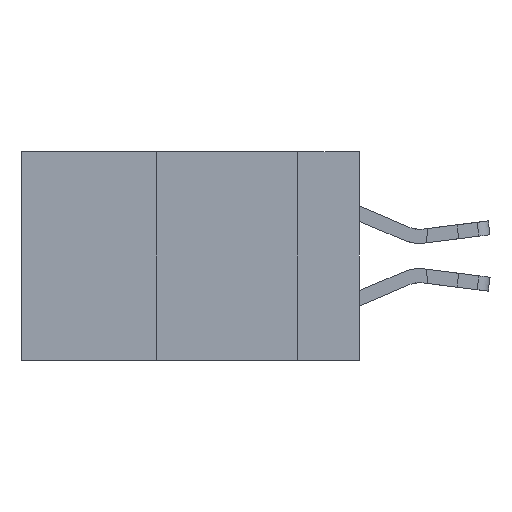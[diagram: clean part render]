
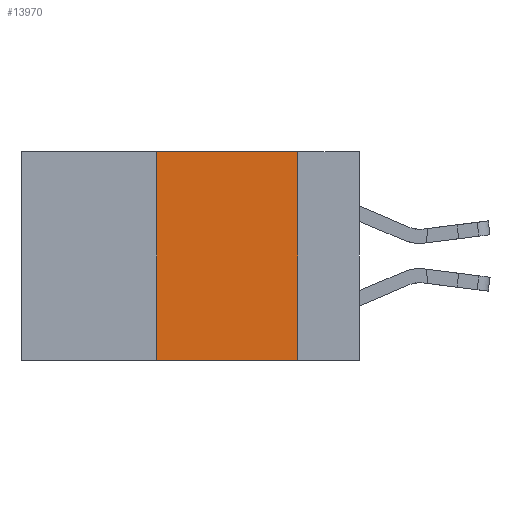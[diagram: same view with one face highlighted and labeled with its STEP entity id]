
A CAD part, left-side view. The second image highlights one B-rep face of the part: STEP entity #13970.
In plain terms, the highlighted planar face has unit normal (-1, 0, 0).
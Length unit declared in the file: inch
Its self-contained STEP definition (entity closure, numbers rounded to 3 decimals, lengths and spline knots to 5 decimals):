
#1781 = ORIENTED_EDGE ( 'NONE', *, *, #9052, .T. ) ;
#1898 = CARTESIAN_POINT ( 'NONE',  ( 0., 0.6, 0. ) ) ;
#2074 = DIRECTION ( 'NONE',  ( 0., 0., -1. ) ) ;
#4413 = DIRECTION ( 'NONE',  ( 0., 0., 1. ) ) ;
#4667 = AXIS2_PLACEMENT_3D ( 'NONE', #1898, #16192, #2074 ) ;
#4872 = VERTEX_POINT ( 'NONE', #6085 ) ;
#5709 = CARTESIAN_POINT ( 'NONE',  ( 0., 0.6, -0.37 ) ) ;
#6085 = CARTESIAN_POINT ( 'NONE',  ( 0., 0.11, -0.37 ) ) ;
#6759 = VECTOR ( 'NONE', #20128, 39.37008 ) ;
#7204 = VERTEX_POINT ( 'NONE', #17203 ) ;
#8339 = FACE_OUTER_BOUND ( 'NONE', #14461, .T. ) ;
#8638 = LINE ( 'NONE', #14356, #6759 ) ;
#9052 = EDGE_CURVE ( 'NONE', #7204, #4872, #20487, .T. ) ;
#9304 = VECTOR ( 'NONE', #25523, 39.37008 ) ;
#10194 = VERTEX_POINT ( 'NONE', #14275 ) ;
#10399 = CARTESIAN_POINT ( 'NONE',  ( 0., 0.36, 0. ) ) ;
#10911 = EDGE_CURVE ( 'NONE', #14034, #10194, #14705, .T. ) ;
#11121 = EDGE_CURVE ( 'NONE', #10194, #4872, #8638, .T. ) ;
#12090 = ORIENTED_EDGE ( 'NONE', *, *, #11121, .F. ) ;
#13970 = ADVANCED_FACE ( 'NONE', ( #8339 ), #17430, .F. ) ;
#14034 = VERTEX_POINT ( 'NONE', #24720 ) ;
#14275 = CARTESIAN_POINT ( 'NONE',  ( 0., 0.11, 0. ) ) ;
#14356 = CARTESIAN_POINT ( 'NONE',  ( 0., 0.11, 0. ) ) ;
#14461 = EDGE_LOOP ( 'NONE', ( #12090, #22399, #19922, #1781 ) ) ;
#14705 = LINE ( 'NONE', #17452, #9304 ) ;
#15505 = EDGE_CURVE ( 'NONE', #7204, #14034, #23799, .T. ) ;
#16192 = DIRECTION ( 'NONE',  ( 1., 0., 0. ) ) ;
#17203 = CARTESIAN_POINT ( 'NONE',  ( 0., 0.36, -0.37 ) ) ;
#17430 = PLANE ( 'NONE',  #4667 ) ;
#17452 = CARTESIAN_POINT ( 'NONE',  ( 0., 0.6, 0. ) ) ;
#17906 = DIRECTION ( 'NONE',  ( 0., -1., 0. ) ) ;
#19922 = ORIENTED_EDGE ( 'NONE', *, *, #15505, .F. ) ;
#20128 = DIRECTION ( 'NONE',  ( 0., 0., -1. ) ) ;
#20487 = LINE ( 'NONE', #5709, #24628 ) ;
#22399 = ORIENTED_EDGE ( 'NONE', *, *, #10911, .F. ) ;
#23799 = LINE ( 'NONE', #10399, #26051 ) ;
#24628 = VECTOR ( 'NONE', #17906, 39.37008 ) ;
#24720 = CARTESIAN_POINT ( 'NONE',  ( 0., 0.36, 0. ) ) ;
#25523 = DIRECTION ( 'NONE',  ( 0., -1., 0. ) ) ;
#26051 = VECTOR ( 'NONE', #4413, 39.37008 ) ;
